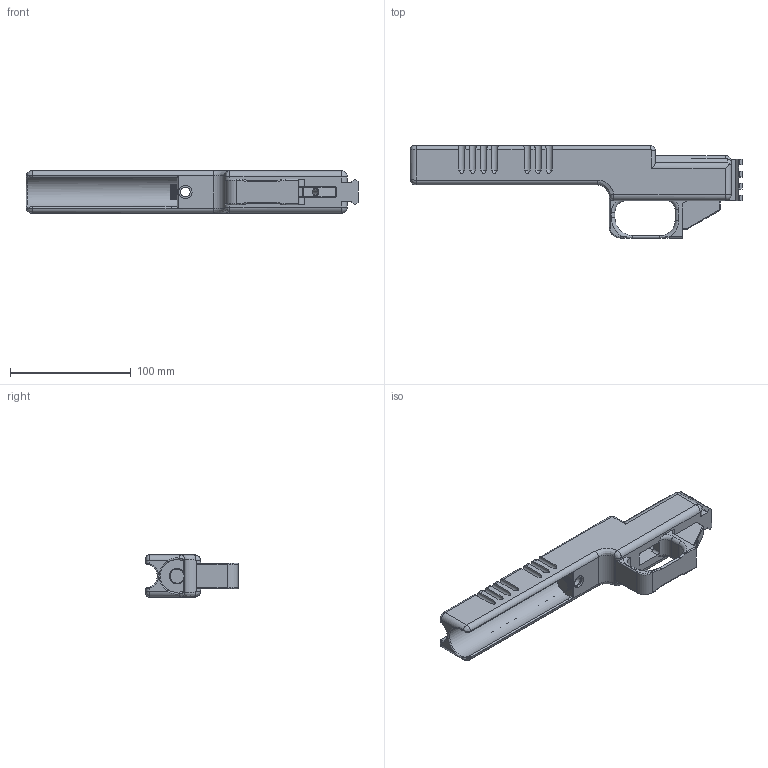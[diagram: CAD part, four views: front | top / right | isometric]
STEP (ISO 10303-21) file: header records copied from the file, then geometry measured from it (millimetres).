
FILE_DESCRIPTION(/* description */ (''),/* implementation_level */ '2;1');
FILE_NAME(/* name */ 'Crickett Chassis Suppressor Mount.step',/* time_stamp */ '2021-04-12T08:37:30-06:00',/* author */ (''),/* organization */ (''),/* preprocessor_version */ 'ST-DEVELOPER v18.1',/* originating_system */ 'Autodesk Translation Framework v10.6.0.1341',/* authorisation */ '');
FILE_SCHEMA (('AUTOMOTIVE_DESIGN { 1 0 10303 214 3 1 1 }'));
Length unit declared in the file: millimetre
Products named in the file (1): Crickett Chassis Suppressor Mount
Bounding box: 274.68 x 76.32 x 35 mm (x, y, z)
Volume: 218112.7 mm3; surface area: 58660.6 mm2
Topology: 1 solids, 1 shells, 322 faces, 893 edges, 557 vertices
Faces by surface type: cylinder 126, plane 122, bspline 36, cone 20, torus 14, sphere 4
Full cylindrical faces by diameter (mm): 8 x1, 11 x1, 11.618 x5, 12.619 x5
Entity records: 13198 total; most frequent: CARTESIAN_POINT 5266, ORIENTED_EDGE 1754, DIRECTION 1528, EDGE_CURVE 877, VERTEX_POINT 557, AXIS2_PLACEMENT_3D 522, LINE 484, VECTOR 484
